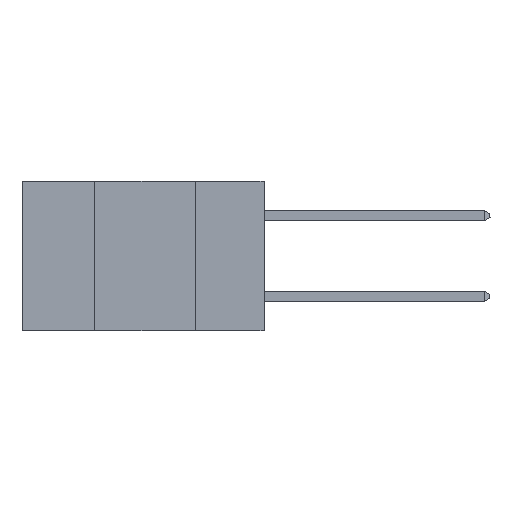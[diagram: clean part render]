
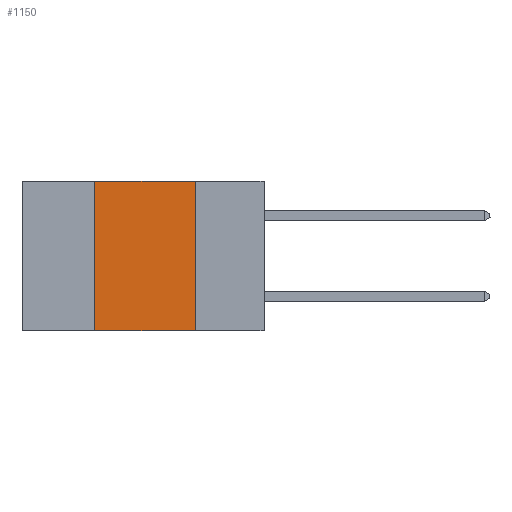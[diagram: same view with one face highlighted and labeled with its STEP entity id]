
A CAD part, left-side view. The second image highlights one B-rep face of the part: STEP entity #1150.
In plain terms, the highlighted planar face has unit normal (-1, 0, 0).
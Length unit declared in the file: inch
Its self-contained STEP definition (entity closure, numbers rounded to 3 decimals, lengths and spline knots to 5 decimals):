
#80 = CARTESIAN_POINT ( 'NONE',  ( 0., 0.17, 0. ) ) ;
#280 = EDGE_CURVE ( 'NONE', #6709, #16469, #4193, .T. ) ;
#298 = EDGE_LOOP ( 'NONE', ( #2675, #15904, #16591, #16084 ) ) ;
#1150 = ADVANCED_FACE ( 'NONE', ( #10391 ), #17119, .F. ) ;
#1687 = VECTOR ( 'NONE', #12729, 39.37008 ) ;
#1947 = CARTESIAN_POINT ( 'NONE',  ( 0., 0.6, 0. ) ) ;
#2675 = ORIENTED_EDGE ( 'NONE', *, *, #12914, .F. ) ;
#2723 = CARTESIAN_POINT ( 'NONE',  ( 0., 0.17, 0. ) ) ;
#3414 = VERTEX_POINT ( 'NONE', #9951 ) ;
#3797 = LINE ( 'NONE', #1947, #1687 ) ;
#3936 = LINE ( 'NONE', #80, #13888 ) ;
#4193 = LINE ( 'NONE', #10271, #7762 ) ;
#5115 = DIRECTION ( 'NONE',  ( 0., 0., 1. ) ) ;
#5117 = DIRECTION ( 'NONE',  ( 1., 0., 0. ) ) ;
#6678 = CARTESIAN_POINT ( 'NONE',  ( 0., 0.17, -0.37 ) ) ;
#6709 = VERTEX_POINT ( 'NONE', #16451 ) ;
#7682 = DIRECTION ( 'NONE',  ( 0., -1., 0. ) ) ;
#7762 = VECTOR ( 'NONE', #7682, 39.37008 ) ;
#8029 = EDGE_CURVE ( 'NONE', #3414, #13897, #3797, .T. ) ;
#9482 = CARTESIAN_POINT ( 'NONE',  ( 0., 0.42, 0. ) ) ;
#9951 = CARTESIAN_POINT ( 'NONE',  ( 0., 0.42, 0. ) ) ;
#10271 = CARTESIAN_POINT ( 'NONE',  ( 0., 0.6, -0.37 ) ) ;
#10339 = DIRECTION ( 'NONE',  ( 0., 0., -1. ) ) ;
#10363 = AXIS2_PLACEMENT_3D ( 'NONE', #10508, #5117, #10339 ) ;
#10391 = FACE_OUTER_BOUND ( 'NONE', #298, .T. ) ;
#10508 = CARTESIAN_POINT ( 'NONE',  ( 0., 0.6, 0. ) ) ;
#10806 = EDGE_CURVE ( 'NONE', #6709, #3414, #14163, .T. ) ;
#12729 = DIRECTION ( 'NONE',  ( 0., -1., 0. ) ) ;
#12914 = EDGE_CURVE ( 'NONE', #13897, #16469, #3936, .T. ) ;
#13247 = DIRECTION ( 'NONE',  ( 0., 0., -1. ) ) ;
#13888 = VECTOR ( 'NONE', #13247, 39.37008 ) ;
#13897 = VERTEX_POINT ( 'NONE', #2723 ) ;
#14163 = LINE ( 'NONE', #9482, #14770 ) ;
#14770 = VECTOR ( 'NONE', #5115, 39.37008 ) ;
#15904 = ORIENTED_EDGE ( 'NONE', *, *, #8029, .F. ) ;
#16084 = ORIENTED_EDGE ( 'NONE', *, *, #280, .T. ) ;
#16451 = CARTESIAN_POINT ( 'NONE',  ( 0., 0.42, -0.37 ) ) ;
#16469 = VERTEX_POINT ( 'NONE', #6678 ) ;
#16591 = ORIENTED_EDGE ( 'NONE', *, *, #10806, .F. ) ;
#17119 = PLANE ( 'NONE',  #10363 ) ;
